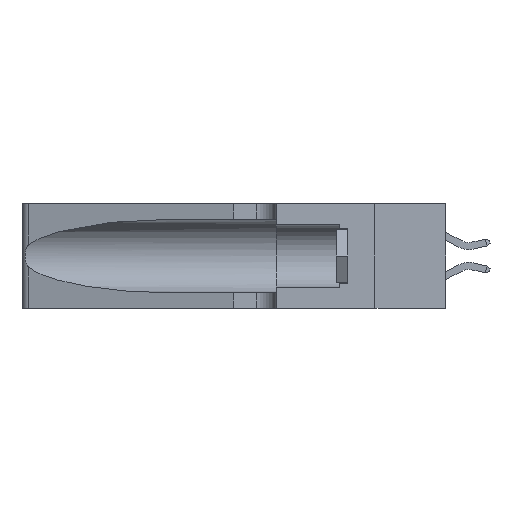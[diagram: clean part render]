
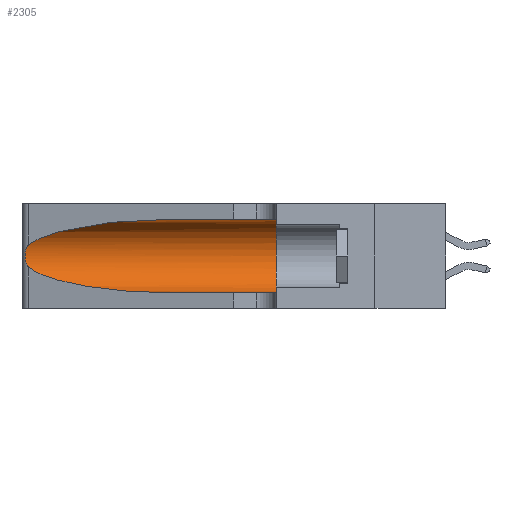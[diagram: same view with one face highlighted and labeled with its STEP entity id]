
A CAD part, left-side view. The second image highlights one B-rep face of the part: STEP entity #2305.
In plain terms, the highlighted cylindrical face has radius 3.308 mm (diameter 6.617 mm), a partial arc.
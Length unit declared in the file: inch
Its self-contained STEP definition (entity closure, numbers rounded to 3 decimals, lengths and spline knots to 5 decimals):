
#194 = CARTESIAN_POINT ( 'NONE',  ( 0.1305, 0.35, 0.31525 ) ) ;
#697 = CARTESIAN_POINT ( 'NONE',  ( 0.1305, 0.72297, 0.31525 ) ) ;
#721 = CARTESIAN_POINT ( 'NONE',  ( 0.1305, 0.72297, 0.05475 ) ) ;
#1835 = CARTESIAN_POINT ( 'NONE',  ( 0.26017, 1.23833, 0.17102 ) ) ;
#1915 = CARTESIAN_POINT ( 'NONE',  ( 0.25854, 1.2359, 0.20912 ) ) ;
#1924 =( BOUNDED_CURVE ( )  B_SPLINE_CURVE ( 3, ( #24760, #7734, #15636, #7807 ),
 .UNSPECIFIED., .F., .F. ) 
 B_SPLINE_CURVE_WITH_KNOTS ( ( 4, 4 ),
 ( 1.5708, 2.84003 ),
 .UNSPECIFIED. ) 
 CURVE ( )  GEOMETRIC_REPRESENTATION_ITEM ( )  RATIONAL_B_SPLINE_CURVE ( ( 1., 0.87, 0.87, 1. ) ) 
 REPRESENTATION_ITEM ( '' )  );
#2001 = CARTESIAN_POINT ( 'NONE',  ( 0.26075, 1.23896, 0.178 ) ) ;
#2303 = EDGE_CURVE ( 'NONE', #8517, #5887, #24711, .T. ) ;
#2305 = ADVANCED_FACE ( 'NONE', ( #7819 ), #15363, .F. ) ;
#3606 = CARTESIAN_POINT ( 'NONE',  ( 0.25555, 1.22993, 0.14849 ) ) ;
#3682 = CARTESIAN_POINT ( 'NONE',  ( 0.26075, 1.23896, 0.19203 ) ) ;
#4374 = DIRECTION ( 'NONE',  ( 0., -1., 0. ) ) ;
#5261 = DIRECTION ( 'NONE',  ( 0., 0., 1. ) ) ;
#5425 = AXIS2_PLACEMENT_3D ( 'NONE', #8318, #19572, #15732 ) ;
#5439 = CARTESIAN_POINT ( 'NONE',  ( 0.25487, 1.22718, 0.14631 ) ) ;
#5757 = VERTEX_POINT ( 'NONE', #194 ) ;
#5887 = VERTEX_POINT ( 'NONE', #8332 ) ;
#6370 = ORIENTED_EDGE ( 'NONE', *, *, #2303, .T. ) ;
#6862 =( BOUNDED_CURVE ( )  B_SPLINE_CURVE ( 3, ( #23964, #16273, #10535, #721 ),
 .UNSPECIFIED., .F., .T. ) 
 B_SPLINE_CURVE_WITH_KNOTS ( ( 4, 4 ),
 ( 3.44316, 4.71239 ),
 .UNSPECIFIED. ) 
 CURVE ( )  GEOMETRIC_REPRESENTATION_ITEM ( )  RATIONAL_B_SPLINE_CURVE ( ( 1., 0.87, 0.87, 1. ) ) 
 REPRESENTATION_ITEM ( '' )  );
#7088 = CARTESIAN_POINT ( 'NONE',  ( 0.1305, 1.61858, 0.31525 ) ) ;
#7660 = CARTESIAN_POINT ( 'NONE',  ( 0.1305, 0.72297, 0.05475 ) ) ;
#7734 = CARTESIAN_POINT ( 'NONE',  ( 0.18966, 0.96281, 0.31525 ) ) ;
#7807 = CARTESIAN_POINT ( 'NONE',  ( 0.25487, 1.22718, 0.22369 ) ) ;
#7819 = FACE_OUTER_BOUND ( 'NONE', #17121, .T. ) ;
#8318 = CARTESIAN_POINT ( 'NONE',  ( 0.1305, 1.61858, 0.185 ) ) ;
#8332 = CARTESIAN_POINT ( 'NONE',  ( 0.1305, 0.35, 0.05475 ) ) ;
#8517 = VERTEX_POINT ( 'NONE', #7660 ) ;
#9370 = VERTEX_POINT ( 'NONE', #697 ) ;
#9729 = EDGE_CURVE ( 'NONE', #9370, #15254, #1924, .T. ) ;
#10424 = LINE ( 'NONE', #7088, #20450 ) ;
#10480 = ORIENTED_EDGE ( 'NONE', *, *, #9729, .T. ) ;
#10535 = CARTESIAN_POINT ( 'NONE',  ( 0.18966, 0.96281, 0.05475 ) ) ;
#10682 = EDGE_CURVE ( 'NONE', #23667, #8517, #6862, .T. ) ;
#11475 = CARTESIAN_POINT ( 'NONE',  ( 0.25639, 1.23184, 0.21858 ) ) ;
#12568 = ORIENTED_EDGE ( 'NONE', *, *, #10682, .T. ) ;
#12646 = CARTESIAN_POINT ( 'NONE',  ( 0.25487, 1.22718, 0.22369 ) ) ;
#12938 = VECTOR ( 'NONE', #4374, 39.37008 ) ;
#12981 = ORIENTED_EDGE ( 'NONE', *, *, #17556, .T. ) ;
#13434 = CARTESIAN_POINT ( 'NONE',  ( 0.25856, 1.23593, 0.16098 ) ) ;
#13488 = B_SPLINE_CURVE_WITH_KNOTS ( 'NONE', 3,
 ( #13515, #18946, #11475, #15211, #1915, #22897, #3682, #2001, #1835, #13434, #17337, #15446, #3606, #17071 ),
 .UNSPECIFIED., .F., .F.,
 ( 4, 2, 2, 2, 2, 2, 4 ),
 ( 0., 0.00027, 0.00053, 0.00107, 0.0016, 0.00187, 0.00214 ),
 .UNSPECIFIED. ) ;
#13515 = CARTESIAN_POINT ( 'NONE',  ( 0.25487, 1.22718, 0.22369 ) ) ;
#14612 = CARTESIAN_POINT ( 'NONE',  ( 0.1305, 0.35, 0.185 ) ) ;
#14864 = DIRECTION ( 'NONE',  ( 0., 1., 0. ) ) ;
#15211 = CARTESIAN_POINT ( 'NONE',  ( 0.25787, 1.23484, 0.2124 ) ) ;
#15254 = VERTEX_POINT ( 'NONE', #12646 ) ;
#15363 = CYLINDRICAL_SURFACE ( 'NONE', #5425, 0.13025 ) ;
#15446 = CARTESIAN_POINT ( 'NONE',  ( 0.25639, 1.23186, 0.15144 ) ) ;
#15636 = CARTESIAN_POINT ( 'NONE',  ( 0.2373, 1.15595, 0.28018 ) ) ;
#15732 = DIRECTION ( 'NONE',  ( 0., 0., -1. ) ) ;
#16273 = CARTESIAN_POINT ( 'NONE',  ( 0.2373, 1.15595, 0.08982 ) ) ;
#16383 = ORIENTED_EDGE ( 'NONE', *, *, #22325, .F. ) ;
#17071 = CARTESIAN_POINT ( 'NONE',  ( 0.25487, 1.22718, 0.14631 ) ) ;
#17121 = EDGE_LOOP ( 'NONE', ( #10480, #12981, #12568, #6370, #16383, #22479 ) ) ;
#17128 = AXIS2_PLACEMENT_3D ( 'NONE', #14612, #14864, #5261 ) ;
#17337 = CARTESIAN_POINT ( 'NONE',  ( 0.25789, 1.23486, 0.15765 ) ) ;
#17556 = EDGE_CURVE ( 'NONE', #15254, #23667, #13488, .T. ) ;
#18553 = EDGE_CURVE ( 'NONE', #9370, #5757, #10424, .T. ) ;
#18946 = CARTESIAN_POINT ( 'NONE',  ( 0.25555, 1.22994, 0.2215 ) ) ;
#19572 = DIRECTION ( 'NONE',  ( 0., -1., 0. ) ) ;
#20450 = VECTOR ( 'NONE', #24382, 39.37008 ) ;
#21452 = CIRCLE ( 'NONE', #17128, 0.13025 ) ;
#21588 = CARTESIAN_POINT ( 'NONE',  ( 0.1305, 1.61858, 0.05475 ) ) ;
#22325 = EDGE_CURVE ( 'NONE', #5757, #5887, #21452, .T. ) ;
#22479 = ORIENTED_EDGE ( 'NONE', *, *, #18553, .F. ) ;
#22897 = CARTESIAN_POINT ( 'NONE',  ( 0.26018, 1.23835, 0.19895 ) ) ;
#23667 = VERTEX_POINT ( 'NONE', #5439 ) ;
#23964 = CARTESIAN_POINT ( 'NONE',  ( 0.25487, 1.22718, 0.14631 ) ) ;
#24382 = DIRECTION ( 'NONE',  ( 0., -1., 0. ) ) ;
#24711 = LINE ( 'NONE', #21588, #12938 ) ;
#24760 = CARTESIAN_POINT ( 'NONE',  ( 0.1305, 0.72297, 0.31525 ) ) ;
